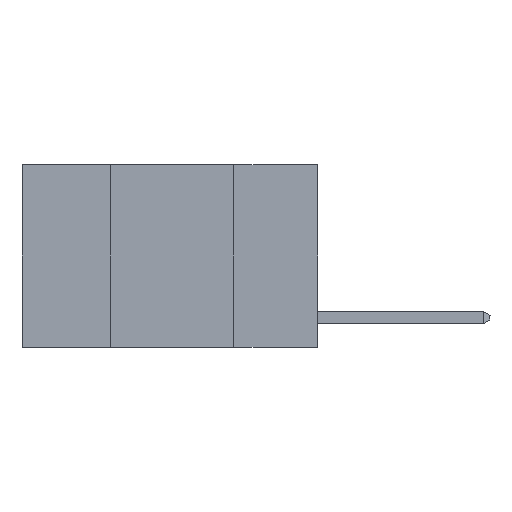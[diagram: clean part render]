
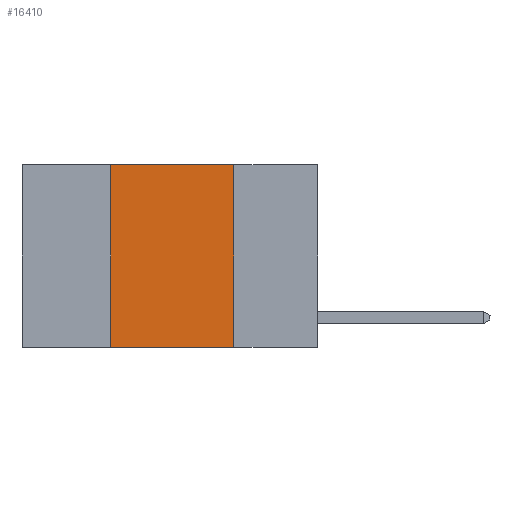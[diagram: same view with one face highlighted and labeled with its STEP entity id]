
A CAD part, left-side view. The second image highlights one B-rep face of the part: STEP entity #16410.
In plain terms, the highlighted planar face has unit normal (-1, 0, 0).
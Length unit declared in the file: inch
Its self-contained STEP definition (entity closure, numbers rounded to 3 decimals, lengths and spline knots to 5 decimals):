
#558 = CARTESIAN_POINT ( 'NONE',  ( 0., 0.6, -0.37 ) ) ;
#1484 = CARTESIAN_POINT ( 'NONE',  ( 0., 0.42, 0. ) ) ;
#1566 = DIRECTION ( 'NONE',  ( 0., 0., 1. ) ) ;
#1844 = DIRECTION ( 'NONE',  ( 1., 0., 0. ) ) ;
#2665 = DIRECTION ( 'NONE',  ( 0., -1., 0. ) ) ;
#2841 = ORIENTED_EDGE ( 'NONE', *, *, #6554, .F. ) ;
#3016 = CARTESIAN_POINT ( 'NONE',  ( 0., 0.17, 0. ) ) ;
#3238 = AXIS2_PLACEMENT_3D ( 'NONE', #14468, #1844, #12972 ) ;
#3487 = FACE_OUTER_BOUND ( 'NONE', #4429, .T. ) ;
#3692 = CARTESIAN_POINT ( 'NONE',  ( 0., 0.17, -0.37 ) ) ;
#4429 = EDGE_LOOP ( 'NONE', ( #2841, #9785, #11945, #16065 ) ) ;
#5127 = VERTEX_POINT ( 'NONE', #3692 ) ;
#5285 = VECTOR ( 'NONE', #1566, 39.37008 ) ;
#6554 = EDGE_CURVE ( 'NONE', #15060, #5127, #9341, .T. ) ;
#8676 = EDGE_CURVE ( 'NONE', #18030, #5127, #14293, .T. ) ;
#8736 = DIRECTION ( 'NONE',  ( 0., -1., 0. ) ) ;
#8910 = PLANE ( 'NONE',  #3238 ) ;
#9341 = LINE ( 'NONE', #17541, #11694 ) ;
#9785 = ORIENTED_EDGE ( 'NONE', *, *, #11891, .F. ) ;
#11478 = CARTESIAN_POINT ( 'NONE',  ( 0., 0.42, 0. ) ) ;
#11694 = VECTOR ( 'NONE', #14965, 39.37008 ) ;
#11891 = EDGE_CURVE ( 'NONE', #15505, #15060, #16776, .T. ) ;
#11945 = ORIENTED_EDGE ( 'NONE', *, *, #16248, .F. ) ;
#11974 = VECTOR ( 'NONE', #2665, 39.37008 ) ;
#12696 = CARTESIAN_POINT ( 'NONE',  ( 0., 0.6, 0. ) ) ;
#12972 = DIRECTION ( 'NONE',  ( 0., 0., -1. ) ) ;
#14197 = LINE ( 'NONE', #1484, #5285 ) ;
#14293 = LINE ( 'NONE', #558, #15463 ) ;
#14449 = CARTESIAN_POINT ( 'NONE',  ( 0., 0.42, -0.37 ) ) ;
#14468 = CARTESIAN_POINT ( 'NONE',  ( 0., 0.6, 0. ) ) ;
#14965 = DIRECTION ( 'NONE',  ( 0., 0., -1. ) ) ;
#15060 = VERTEX_POINT ( 'NONE', #3016 ) ;
#15463 = VECTOR ( 'NONE', #8736, 39.37008 ) ;
#15505 = VERTEX_POINT ( 'NONE', #11478 ) ;
#16065 = ORIENTED_EDGE ( 'NONE', *, *, #8676, .T. ) ;
#16248 = EDGE_CURVE ( 'NONE', #18030, #15505, #14197, .T. ) ;
#16410 = ADVANCED_FACE ( 'NONE', ( #3487 ), #8910, .F. ) ;
#16776 = LINE ( 'NONE', #12696, #11974 ) ;
#17541 = CARTESIAN_POINT ( 'NONE',  ( 0., 0.17, 0. ) ) ;
#18030 = VERTEX_POINT ( 'NONE', #14449 ) ;
